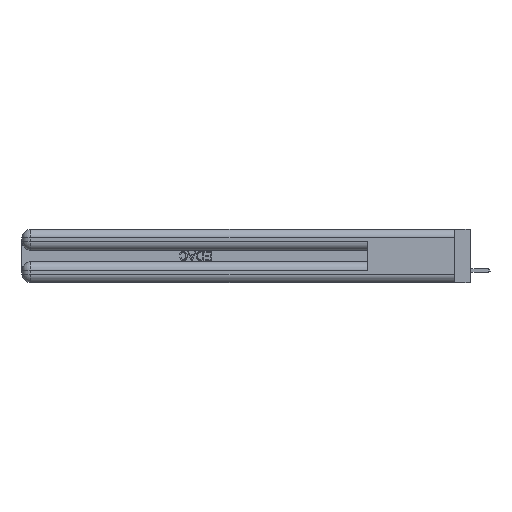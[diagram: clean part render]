
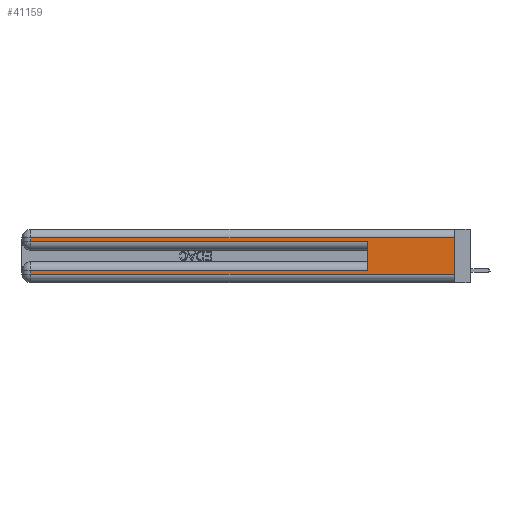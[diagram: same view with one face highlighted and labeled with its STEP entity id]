
A CAD part, left-side view. The second image highlights one B-rep face of the part: STEP entity #41159.
In plain terms, the highlighted planar face has unit normal (-1, 0, 0).
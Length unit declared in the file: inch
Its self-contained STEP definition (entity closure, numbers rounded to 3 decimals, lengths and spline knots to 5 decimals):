
#753 = CARTESIAN_POINT ( 'NONE',  ( 0., 0., 0.37 ) ) ;
#1159 = LINE ( 'NONE', #1506, #37184 ) ;
#1506 = CARTESIAN_POINT ( 'NONE',  ( 0., 0., 0.31 ) ) ;
#1639 = CARTESIAN_POINT ( 'NONE',  ( 0., 0., 0.285 ) ) ;
#1815 = DIRECTION ( 'NONE',  ( 0., -1., 0. ) ) ;
#2019 = FACE_OUTER_BOUND ( 'NONE', #45795, .T. ) ;
#2097 = AXIS2_PLACEMENT_3D ( 'NONE', #27687, #43415, #43765 ) ;
#2122 = EDGE_CURVE ( 'NONE', #36634, #37968, #36267, .T. ) ;
#4184 = VERTEX_POINT ( 'NONE', #30962 ) ;
#4293 = VERTEX_POINT ( 'NONE', #30497 ) ;
#4379 = LINE ( 'NONE', #29379, #40393 ) ;
#4455 = LINE ( 'NONE', #34245, #13831 ) ;
#4514 = DIRECTION ( 'NONE',  ( 0., 0., -1. ) ) ;
#4532 = DIRECTION ( 'NONE',  ( 0., 0., -1. ) ) ;
#5138 = ORIENTED_EDGE ( 'NONE', *, *, #30510, .T. ) ;
#5228 = ORIENTED_EDGE ( 'NONE', *, *, #34809, .T. ) ;
#9347 = DIRECTION ( 'NONE',  ( 0., 1., 0. ) ) ;
#9728 = CARTESIAN_POINT ( 'NONE',  ( 0., 2.94, 0.06 ) ) ;
#10055 = DIRECTION ( 'NONE',  ( 0., 1., 0. ) ) ;
#10667 = DIRECTION ( 'NONE',  ( 0., 0., -1. ) ) ;
#10915 = ORIENTED_EDGE ( 'NONE', *, *, #27387, .T. ) ;
#11916 = CARTESIAN_POINT ( 'NONE',  ( 0., 2.94, 0.37 ) ) ;
#13128 = ORIENTED_EDGE ( 'NONE', *, *, #2122, .F. ) ;
#13299 = LINE ( 'NONE', #11916, #20897 ) ;
#13350 = ORIENTED_EDGE ( 'NONE', *, *, #49291, .T. ) ;
#13831 = VECTOR ( 'NONE', #10055, 39.37008 ) ;
#14272 = CARTESIAN_POINT ( 'NONE',  ( 0., 0.6, 0.085 ) ) ;
#16312 = VERTEX_POINT ( 'NONE', #30790 ) ;
#19082 = ORIENTED_EDGE ( 'NONE', *, *, #34721, .T. ) ;
#19842 = CARTESIAN_POINT ( 'NONE',  ( 0., 0., 0.06 ) ) ;
#20047 = CARTESIAN_POINT ( 'NONE',  ( 0., 0.6, 0.145 ) ) ;
#20897 = VECTOR ( 'NONE', #4514, 39.37008 ) ;
#25718 = LINE ( 'NONE', #753, #51136 ) ;
#27387 = EDGE_CURVE ( 'NONE', #31712, #4184, #13299, .T. ) ;
#27687 = CARTESIAN_POINT ( 'NONE',  ( 0., 0., 0.37 ) ) ;
#27821 = ORIENTED_EDGE ( 'NONE', *, *, #36988, .T. ) ;
#29379 = CARTESIAN_POINT ( 'NONE',  ( 0., 0., 0.06 ) ) ;
#29549 = VECTOR ( 'NONE', #10667, 39.37008 ) ;
#30497 = CARTESIAN_POINT ( 'NONE',  ( 0., 2.94, 0.085 ) ) ;
#30510 = EDGE_CURVE ( 'NONE', #4184, #37968, #39555, .T. ) ;
#30790 = CARTESIAN_POINT ( 'NONE',  ( 0., 0., 0.31 ) ) ;
#30962 = CARTESIAN_POINT ( 'NONE',  ( 0., 2.94, 0.285 ) ) ;
#31712 = VERTEX_POINT ( 'NONE', #35260 ) ;
#32440 = VERTEX_POINT ( 'NONE', #9728 ) ;
#34245 = CARTESIAN_POINT ( 'NONE',  ( 0., 0., 0.085 ) ) ;
#34721 = EDGE_CURVE ( 'NONE', #32440, #50148, #4379, .T. ) ;
#34809 = EDGE_CURVE ( 'NONE', #16312, #31712, #1159, .T. ) ;
#35260 = CARTESIAN_POINT ( 'NONE',  ( 0., 2.94, 0.31 ) ) ;
#36010 = DIRECTION ( 'NONE',  ( 0., 0., 1. ) ) ;
#36267 = LINE ( 'NONE', #20047, #40090 ) ;
#36634 = VERTEX_POINT ( 'NONE', #14272 ) ;
#36988 = EDGE_CURVE ( 'NONE', #4293, #32440, #47306, .T. ) ;
#37184 = VECTOR ( 'NONE', #9347, 39.37008 ) ;
#37968 = VERTEX_POINT ( 'NONE', #48804 ) ;
#39555 = LINE ( 'NONE', #1639, #46482 ) ;
#40090 = VECTOR ( 'NONE', #36010, 39.37008 ) ;
#40393 = VECTOR ( 'NONE', #46514, 39.37008 ) ;
#41159 = ADVANCED_FACE ( 'NONE', ( #2019 ), #47121, .F. ) ;
#43415 = DIRECTION ( 'NONE',  ( 1., 0., 0. ) ) ;
#43765 = DIRECTION ( 'NONE',  ( 0., 0., -1. ) ) ;
#45795 = EDGE_LOOP ( 'NONE', ( #50132, #5228, #10915, #5138, #13128, #13350, #27821, #19082 ) ) ;
#46482 = VECTOR ( 'NONE', #1815, 39.37008 ) ;
#46514 = DIRECTION ( 'NONE',  ( 0., -1., 0. ) ) ;
#47121 = PLANE ( 'NONE',  #2097 ) ;
#47306 = LINE ( 'NONE', #50645, #29549 ) ;
#48804 = CARTESIAN_POINT ( 'NONE',  ( 0., 0.6, 0.285 ) ) ;
#49291 = EDGE_CURVE ( 'NONE', #36634, #4293, #4455, .T. ) ;
#50132 = ORIENTED_EDGE ( 'NONE', *, *, #50380, .F. ) ;
#50148 = VERTEX_POINT ( 'NONE', #19842 ) ;
#50380 = EDGE_CURVE ( 'NONE', #16312, #50148, #25718, .T. ) ;
#50645 = CARTESIAN_POINT ( 'NONE',  ( 0., 2.94, 0.37 ) ) ;
#51136 = VECTOR ( 'NONE', #4532, 39.37008 ) ;
